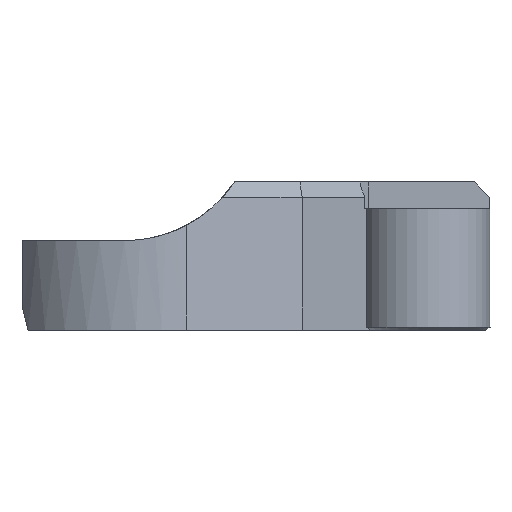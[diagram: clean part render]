
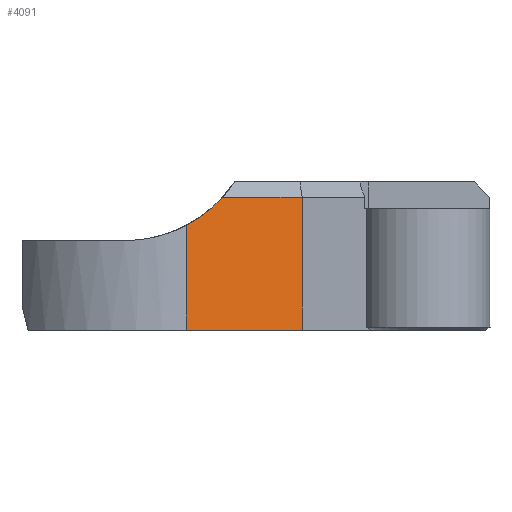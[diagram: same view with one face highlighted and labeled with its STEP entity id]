
A CAD part, front view. The second image highlights one B-rep face of the part: STEP entity #4091.
In plain terms, the highlighted planar face has unit normal (0.279, -0.96, 0).
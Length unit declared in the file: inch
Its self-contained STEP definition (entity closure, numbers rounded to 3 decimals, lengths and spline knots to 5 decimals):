
#27 = VERTEX_POINT ( 'NONE', #1758 ) ;
#266 = EDGE_CURVE ( 'NONE', #6804, #4927, #466, .T. ) ;
#466 = LINE ( 'NONE', #7372, #6182 ) ;
#506 = CARTESIAN_POINT ( 'NONE',  ( 3.07817, -0.37391, 4.00548 ) ) ;
#1373 = ORIENTED_EDGE ( 'NONE', *, *, #4124, .F. ) ;
#1758 = CARTESIAN_POINT ( 'NONE',  ( 2.87502, -0.43289, 3.84899 ) ) ;
#1947 = DIRECTION ( 'NONE',  ( -0.96, -0.279, 0. ) ) ;
#2010 = CARTESIAN_POINT ( 'NONE',  ( 2.87502, -0.43289, 3.84899 ) ) ;
#2490 = ORIENTED_EDGE ( 'NONE', *, *, #266, .T. ) ;
#2576 = CARTESIAN_POINT ( 'NONE',  ( 2.95141, -0.41071, 3.8892 ) ) ;
#2741 = CARTESIAN_POINT ( 'NONE',  ( 3.52564, -0.24399, 6.36544 ) ) ;
#3079 = DIRECTION ( 'NONE',  ( 0., 0., -1. ) ) ;
#3101 = ORIENTED_EDGE ( 'NONE', *, *, #5266, .F. ) ;
#3355 = AXIS2_PLACEMENT_3D ( 'NONE', #2741, #4513, #7029 ) ;
#3361 = CARTESIAN_POINT ( 'NONE',  ( 3.52564, -0.24399, 3.25964 ) ) ;
#4061 = CARTESIAN_POINT ( 'NONE',  ( 3.52564, -0.24399, 6.36544 ) ) ;
#4091 = ADVANCED_FACE ( 'NONE', ( #5034 ), #5785, .T. ) ;
#4124 = EDGE_CURVE ( 'NONE', #4151, #6261, #7323, .T. ) ;
#4151 = VERTEX_POINT ( 'NONE', #6028 ) ;
#4194 = VECTOR ( 'NONE', #5883, 39.37008 ) ;
#4428 = EDGE_CURVE ( 'NONE', #27, #6261, #6454, .T. ) ;
#4513 = DIRECTION ( 'NONE',  ( 0.279, -0.96, 0. ) ) ;
#4549 = CARTESIAN_POINT ( 'NONE',  ( 3.52564, -0.24399, 4.00548 ) ) ;
#4571 = ORIENTED_EDGE ( 'NONE', *, *, #4428, .T. ) ;
#4579 = LINE ( 'NONE', #4061, #4194 ) ;
#4689 = EDGE_LOOP ( 'NONE', ( #6721, #2490, #3101, #4571, #1373 ) ) ;
#4927 = VERTEX_POINT ( 'NONE', #506 ) ;
#5034 = FACE_OUTER_BOUND ( 'NONE', #4689, .T. ) ;
#5212 = DIRECTION ( 'NONE',  ( -0.96, -0.279, 0. ) ) ;
#5266 = EDGE_CURVE ( 'NONE', #27, #4927, #6240, .T. ) ;
#5416 = VECTOR ( 'NONE', #5212, 39.37008 ) ;
#5785 = PLANE ( 'NONE',  #3355 ) ;
#5883 = DIRECTION ( 'NONE',  ( 0., 0., -1. ) ) ;
#6028 = CARTESIAN_POINT ( 'NONE',  ( 3.52564, -0.24399, 3.25964 ) ) ;
#6125 = EDGE_CURVE ( 'NONE', #6804, #4151, #4579, .T. ) ;
#6182 = VECTOR ( 'NONE', #1947, 39.37008 ) ;
#6235 = CARTESIAN_POINT ( 'NONE',  ( 3.01979, -0.39086, 3.94188 ) ) ;
#6240 =( BOUNDED_CURVE ( )  B_SPLINE_CURVE ( 3, ( #2010, #2576, #6235, #7413 ),
 .UNSPECIFIED., .F., .F. ) 
 B_SPLINE_CURVE_WITH_KNOTS ( ( 4, 4 ),
 ( 5.19698, 5.54056 ),
 .UNSPECIFIED. ) 
 CURVE ( )  GEOMETRIC_REPRESENTATION_ITEM ( )  RATIONAL_B_SPLINE_CURVE ( ( 1., 0.99, 0.99, 1. ) ) 
 REPRESENTATION_ITEM ( '' )  );
#6261 = VERTEX_POINT ( 'NONE', #7340 ) ;
#6357 = VECTOR ( 'NONE', #3079, 39.37008 ) ;
#6454 = LINE ( 'NONE', #6738, #6357 ) ;
#6721 = ORIENTED_EDGE ( 'NONE', *, *, #6125, .F. ) ;
#6738 = CARTESIAN_POINT ( 'NONE',  ( 2.87502, -0.43289, 6.36544 ) ) ;
#6804 = VERTEX_POINT ( 'NONE', #4549 ) ;
#7029 = DIRECTION ( 'NONE',  ( -0.96, -0.279, 0. ) ) ;
#7323 = LINE ( 'NONE', #3361, #5416 ) ;
#7340 = CARTESIAN_POINT ( 'NONE',  ( 2.87502, -0.43289, 3.25964 ) ) ;
#7372 = CARTESIAN_POINT ( 'NONE',  ( 3.14724, -0.35385, 4.00548 ) ) ;
#7413 = CARTESIAN_POINT ( 'NONE',  ( 3.07817, -0.37391, 4.00548 ) ) ;
